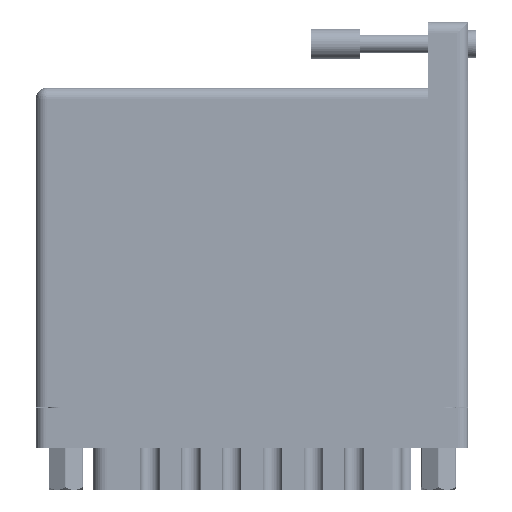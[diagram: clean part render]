
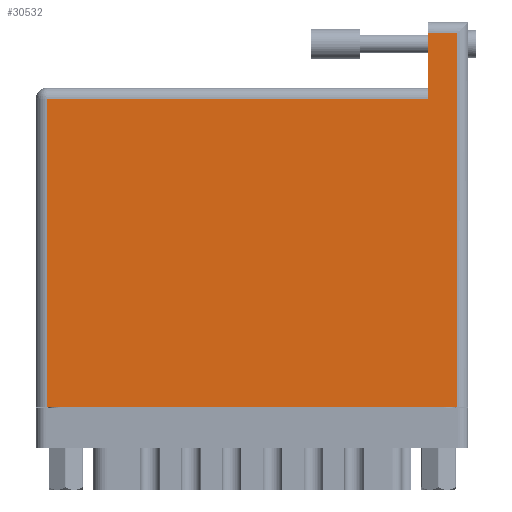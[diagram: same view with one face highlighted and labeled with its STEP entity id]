
A CAD part, front view. The second image highlights one B-rep face of the part: STEP entity #30532.
In plain terms, the highlighted face is planar.
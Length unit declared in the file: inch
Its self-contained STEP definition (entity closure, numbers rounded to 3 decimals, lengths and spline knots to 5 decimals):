
#3232 = EDGE_CURVE ( 'NONE', #30434, #11083, #47125, .T. ) ;
#5532 = ORIENTED_EDGE ( 'NONE', *, *, #71689, .T. ) ;
#6266 = LINE ( 'NONE', #52364, #44542 ) ;
#11083 = VERTEX_POINT ( 'NONE', #12419 ) ;
#12256 = EDGE_LOOP ( 'NONE', ( #14077, #105226, #26562, #18325, #5532, #48717 ) ) ;
#12419 = CARTESIAN_POINT ( 'NONE',  ( 2.499, 1.96, 0. ) ) ;
#14077 = ORIENTED_EDGE ( 'NONE', *, *, #3232, .T. ) ;
#15641 = CARTESIAN_POINT ( 'NONE',  ( 2.685, 2.38, 0. ) ) ;
#16603 = VECTOR ( 'NONE', #47030, 39.37008 ) ;
#18325 = ORIENTED_EDGE ( 'NONE', *, *, #28694, .T. ) ;
#19558 = DIRECTION ( 'NONE',  ( 1., 0., 0. ) ) ;
#21192 = DIRECTION ( 'NONE',  ( 0., 1., 0. ) ) ;
#21427 = EDGE_CURVE ( 'NONE', #58119, #105645, #6266, .T. ) ;
#26562 = ORIENTED_EDGE ( 'NONE', *, *, #21427, .T. ) ;
#28223 = CARTESIAN_POINT ( 'NONE',  ( 0.07, 0., 0. ) ) ;
#28641 = VECTOR ( 'NONE', #55376, 39.37008 ) ;
#28694 = EDGE_CURVE ( 'NONE', #105645, #83908, #48075, .T. ) ;
#30434 = VERTEX_POINT ( 'NONE', #68327 ) ;
#30532 = ADVANCED_FACE ( 'NONE', ( #42305 ), #36228, .F. ) ;
#36228 = PLANE ( 'NONE',  #73770 ) ;
#39179 = VECTOR ( 'NONE', #19558, 39.37008 ) ;
#39463 = VECTOR ( 'NONE', #56298, 39.37008 ) ;
#42305 = FACE_OUTER_BOUND ( 'NONE', #12256, .T. ) ;
#44454 = DIRECTION ( 'NONE',  ( 0., 0., -1. ) ) ;
#44542 = VECTOR ( 'NONE', #68526, 39.37008 ) ;
#44805 = DIRECTION ( 'NONE',  ( -1., 0., 0. ) ) ;
#47030 = DIRECTION ( 'NONE',  ( -1., 0., 0. ) ) ;
#47125 = LINE ( 'NONE', #48805, #39463 ) ;
#48075 = LINE ( 'NONE', #60874, #39179 ) ;
#48717 = ORIENTED_EDGE ( 'NONE', *, *, #79663, .T. ) ;
#48805 = CARTESIAN_POINT ( 'NONE',  ( 2.499, 2.45, 0. ) ) ;
#52364 = CARTESIAN_POINT ( 'NONE',  ( 0.07, 0., 0. ) ) ;
#54247 = EDGE_CURVE ( 'NONE', #11083, #58119, #83034, .T. ) ;
#55376 = DIRECTION ( 'NONE',  ( -1., 0., 0. ) ) ;
#56298 = DIRECTION ( 'NONE',  ( 0., -1., 0. ) ) ;
#58119 = VERTEX_POINT ( 'NONE', #65424 ) ;
#60874 = CARTESIAN_POINT ( 'NONE',  ( 0., 0., 0. ) ) ;
#61070 = VERTEX_POINT ( 'NONE', #15641 ) ;
#64090 = CARTESIAN_POINT ( 'NONE',  ( 0., 1.96, 0. ) ) ;
#65424 = CARTESIAN_POINT ( 'NONE',  ( 0.07, 1.96, 0. ) ) ;
#67068 = VECTOR ( 'NONE', #21192, 39.37008 ) ;
#68327 = CARTESIAN_POINT ( 'NONE',  ( 2.499, 2.38, 0. ) ) ;
#68526 = DIRECTION ( 'NONE',  ( 0., -1., 0. ) ) ;
#71689 = EDGE_CURVE ( 'NONE', #83908, #61070, #94112, .T. ) ;
#73770 = AXIS2_PLACEMENT_3D ( 'NONE', #93481, #44454, #44805 ) ;
#79663 = EDGE_CURVE ( 'NONE', #61070, #30434, #95271, .T. ) ;
#83034 = LINE ( 'NONE', #64090, #16603 ) ;
#83908 = VERTEX_POINT ( 'NONE', #104585 ) ;
#85515 = CARTESIAN_POINT ( 'NONE',  ( 2.685, 2.45, 0. ) ) ;
#93481 = CARTESIAN_POINT ( 'NONE',  ( 0., 2.03, 0. ) ) ;
#94112 = LINE ( 'NONE', #85515, #67068 ) ;
#95271 = LINE ( 'NONE', #96242, #28641 ) ;
#96242 = CARTESIAN_POINT ( 'NONE',  ( 0., 2.38, 0. ) ) ;
#104585 = CARTESIAN_POINT ( 'NONE',  ( 2.685, 0., 0. ) ) ;
#105226 = ORIENTED_EDGE ( 'NONE', *, *, #54247, .T. ) ;
#105645 = VERTEX_POINT ( 'NONE', #28223 ) ;
